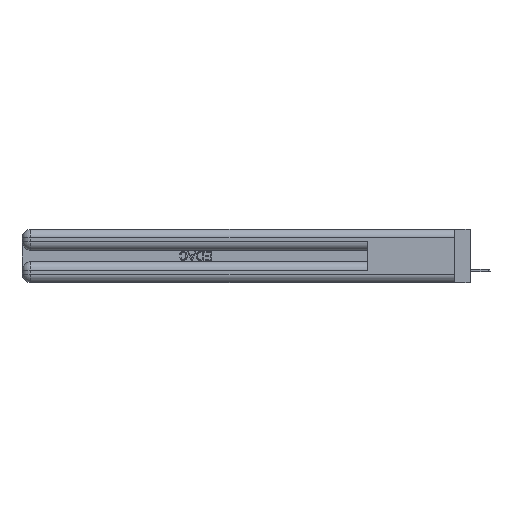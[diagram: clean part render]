
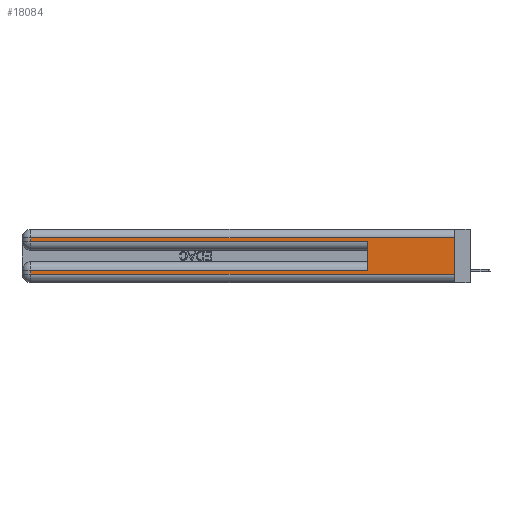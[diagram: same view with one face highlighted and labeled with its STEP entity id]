
A CAD part, left-side view. The second image highlights one B-rep face of the part: STEP entity #18084.
In plain terms, the highlighted planar face has unit normal (-1, 0, 0).
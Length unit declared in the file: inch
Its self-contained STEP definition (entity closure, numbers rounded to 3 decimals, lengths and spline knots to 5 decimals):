
#1160 = VERTEX_POINT ( 'NONE', #36501 ) ;
#1303 = VECTOR ( 'NONE', #27605, 39.37008 ) ;
#1894 = DIRECTION ( 'NONE',  ( 0., 1., 0. ) ) ;
#2051 = VERTEX_POINT ( 'NONE', #8106 ) ;
#2457 = VECTOR ( 'NONE', #11905, 39.37008 ) ;
#2887 = VERTEX_POINT ( 'NONE', #31952 ) ;
#5731 = CARTESIAN_POINT ( 'NONE',  ( 0., 0., 0.31 ) ) ;
#6187 = CARTESIAN_POINT ( 'NONE',  ( 0., 0.6, 0.285 ) ) ;
#6337 = VERTEX_POINT ( 'NONE', #44923 ) ;
#7956 = ORIENTED_EDGE ( 'NONE', *, *, #8749, .T. ) ;
#7969 = FACE_OUTER_BOUND ( 'NONE', #35369, .T. ) ;
#8106 = CARTESIAN_POINT ( 'NONE',  ( 0., 2.94, 0.085 ) ) ;
#8203 = CARTESIAN_POINT ( 'NONE',  ( 0., 0., 0.37 ) ) ;
#8749 = EDGE_CURVE ( 'NONE', #41480, #38830, #16486, .T. ) ;
#9371 = EDGE_CURVE ( 'NONE', #2051, #15513, #37897, .T. ) ;
#9750 = CARTESIAN_POINT ( 'NONE',  ( 0., 2.94, 0.285 ) ) ;
#10942 = DIRECTION ( 'NONE',  ( 0., 0., -1. ) ) ;
#11905 = DIRECTION ( 'NONE',  ( 0., 1., 0. ) ) ;
#12002 = VECTOR ( 'NONE', #38720, 39.37008 ) ;
#12120 = LINE ( 'NONE', #5731, #32294 ) ;
#14159 = CARTESIAN_POINT ( 'NONE',  ( 0., 2.94, 0.37 ) ) ;
#15038 = CARTESIAN_POINT ( 'NONE',  ( 0., 2.94, 0.37 ) ) ;
#15453 = VERTEX_POINT ( 'NONE', #38252 ) ;
#15513 = VERTEX_POINT ( 'NONE', #21776 ) ;
#15587 = ORIENTED_EDGE ( 'NONE', *, *, #36293, .T. ) ;
#16486 = LINE ( 'NONE', #29336, #20146 ) ;
#17247 = ORIENTED_EDGE ( 'NONE', *, *, #19236, .T. ) ;
#17480 = LINE ( 'NONE', #24320, #12002 ) ;
#17858 = EDGE_CURVE ( 'NONE', #6337, #15453, #12120, .T. ) ;
#18084 = ADVANCED_FACE ( 'NONE', ( #7969 ), #21437, .F. ) ;
#19236 = EDGE_CURVE ( 'NONE', #15453, #41480, #39688, .T. ) ;
#20146 = VECTOR ( 'NONE', #30402, 39.37008 ) ;
#21170 = VECTOR ( 'NONE', #40566, 39.37008 ) ;
#21223 = DIRECTION ( 'NONE',  ( 1., 0., 0. ) ) ;
#21423 = VECTOR ( 'NONE', #21886, 39.37008 ) ;
#21437 = PLANE ( 'NONE',  #41039 ) ;
#21776 = CARTESIAN_POINT ( 'NONE',  ( 0., 2.94, 0.06 ) ) ;
#21886 = DIRECTION ( 'NONE',  ( 0., 0., -1. ) ) ;
#22015 = ORIENTED_EDGE ( 'NONE', *, *, #9371, .T. ) ;
#22524 = ORIENTED_EDGE ( 'NONE', *, *, #34571, .T. ) ;
#22770 = CARTESIAN_POINT ( 'NONE',  ( 0., 0., 0.37 ) ) ;
#23637 = ORIENTED_EDGE ( 'NONE', *, *, #17858, .T. ) ;
#24205 = EDGE_CURVE ( 'NONE', #6337, #2887, #36915, .T. ) ;
#24320 = CARTESIAN_POINT ( 'NONE',  ( 0., 0., 0.06 ) ) ;
#24474 = LINE ( 'NONE', #34768, #43753 ) ;
#25802 = CARTESIAN_POINT ( 'NONE',  ( 0., 0., 0.085 ) ) ;
#25884 = ORIENTED_EDGE ( 'NONE', *, *, #44553, .F. ) ;
#27405 = ORIENTED_EDGE ( 'NONE', *, *, #24205, .F. ) ;
#27605 = DIRECTION ( 'NONE',  ( 0., 0., -1. ) ) ;
#29336 = CARTESIAN_POINT ( 'NONE',  ( 0., 0., 0.285 ) ) ;
#30402 = DIRECTION ( 'NONE',  ( 0., -1., 0. ) ) ;
#31952 = CARTESIAN_POINT ( 'NONE',  ( 0., 0., 0.06 ) ) ;
#32294 = VECTOR ( 'NONE', #1894, 39.37008 ) ;
#32662 = LINE ( 'NONE', #25802, #2457 ) ;
#34571 = EDGE_CURVE ( 'NONE', #1160, #2051, #32662, .T. ) ;
#34768 = CARTESIAN_POINT ( 'NONE',  ( 0., 0.6, 0.145 ) ) ;
#35369 = EDGE_LOOP ( 'NONE', ( #27405, #23637, #17247, #7956, #25884, #22524, #22015, #15587 ) ) ;
#36293 = EDGE_CURVE ( 'NONE', #15513, #2887, #17480, .T. ) ;
#36501 = CARTESIAN_POINT ( 'NONE',  ( 0., 0.6, 0.085 ) ) ;
#36915 = LINE ( 'NONE', #22770, #21170 ) ;
#37897 = LINE ( 'NONE', #14159, #1303 ) ;
#38252 = CARTESIAN_POINT ( 'NONE',  ( 0., 2.94, 0.31 ) ) ;
#38720 = DIRECTION ( 'NONE',  ( 0., -1., 0. ) ) ;
#38830 = VERTEX_POINT ( 'NONE', #6187 ) ;
#39688 = LINE ( 'NONE', #15038, #21423 ) ;
#40566 = DIRECTION ( 'NONE',  ( 0., 0., -1. ) ) ;
#41039 = AXIS2_PLACEMENT_3D ( 'NONE', #8203, #21223, #10942 ) ;
#41480 = VERTEX_POINT ( 'NONE', #9750 ) ;
#43753 = VECTOR ( 'NONE', #45037, 39.37008 ) ;
#44553 = EDGE_CURVE ( 'NONE', #1160, #38830, #24474, .T. ) ;
#44923 = CARTESIAN_POINT ( 'NONE',  ( 0., 0., 0.31 ) ) ;
#45037 = DIRECTION ( 'NONE',  ( 0., 0., 1. ) ) ;
